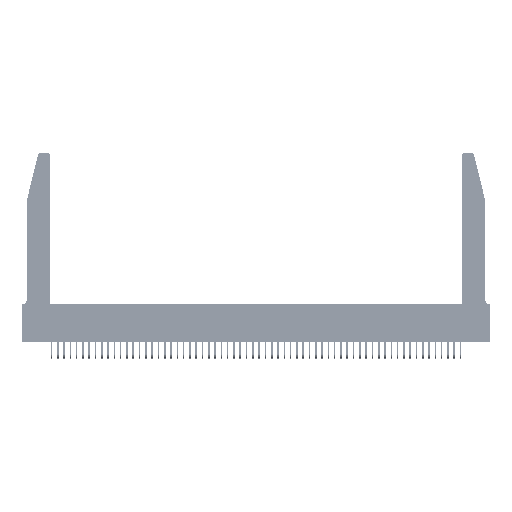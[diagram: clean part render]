
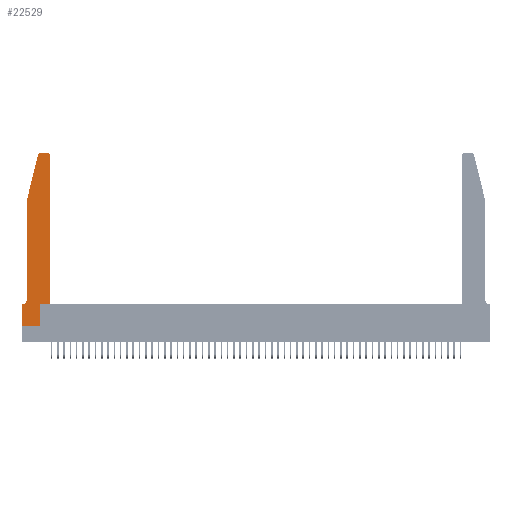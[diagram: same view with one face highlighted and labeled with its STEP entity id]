
A CAD part, top view. The second image highlights one B-rep face of the part: STEP entity #22529.
In plain terms, the highlighted planar face has unit normal (0, 0, 1).
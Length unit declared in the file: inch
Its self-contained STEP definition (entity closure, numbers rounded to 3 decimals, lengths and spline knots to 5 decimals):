
#350 = VECTOR ( 'NONE', #27360, 39.37008 ) ;
#563 = CARTESIAN_POINT ( 'NONE',  ( 0.0755, 0.42, 0.37 ) ) ;
#987 = DIRECTION ( 'NONE',  ( 0., -1., 0. ) ) ;
#1433 = VECTOR ( 'NONE', #987, 39.37008 ) ;
#1503 = CARTESIAN_POINT ( 'NONE',  ( 0.2865, 0., 0.37 ) ) ;
#2649 = CARTESIAN_POINT ( 'NONE',  ( 0., 0., 0.37 ) ) ;
#2734 = CARTESIAN_POINT ( 'NONE',  ( 0.284, 2.72, 0.37 ) ) ;
#3942 = DIRECTION ( 'NONE',  ( 0., 0., 1. ) ) ;
#4755 = ORIENTED_EDGE ( 'NONE', *, *, #19463, .T. ) ;
#5805 = EDGE_CURVE ( 'NONE', #31619, #9378, #43593, .T. ) ;
#7112 = DIRECTION ( 'NONE',  ( 1., 0., 0. ) ) ;
#7385 = EDGE_CURVE ( 'NONE', #28030, #43568, #21678, .T. ) ;
#7864 = EDGE_CURVE ( 'NONE', #11868, #31619, #13019, .T. ) ;
#9285 = LINE ( 'NONE', #33301, #50271 ) ;
#9378 = VERTEX_POINT ( 'NONE', #27630 ) ;
#10865 = CIRCLE ( 'NONE', #11652, 0.03 ) ;
#11652 = AXIS2_PLACEMENT_3D ( 'NONE', #23470, #52870, #27705 ) ;
#11660 = EDGE_CURVE ( 'NONE', #17356, #39878, #17730, .T. ) ;
#11868 = VERTEX_POINT ( 'NONE', #22654 ) ;
#12125 = VECTOR ( 'NONE', #21281, 39.37008 ) ;
#12420 = VECTOR ( 'NONE', #38266, 39.37008 ) ;
#12501 = PLANE ( 'NONE',  #33237 ) ;
#12825 = CARTESIAN_POINT ( 'NONE',  ( 0.0055, 0.42, 0.37 ) ) ;
#12856 = DIRECTION ( 'NONE',  ( 1., 0., 0. ) ) ;
#13019 = LINE ( 'NONE', #30898, #1433 ) ;
#13197 = EDGE_CURVE ( 'NONE', #49335, #43265, #10865, .T. ) ;
#13372 = ORIENTED_EDGE ( 'NONE', *, *, #11660, .T. ) ;
#16410 = VECTOR ( 'NONE', #12856, 39.37008 ) ;
#16465 = CARTESIAN_POINT ( 'NONE',  ( 0.4205, 2.75, 0.37 ) ) ;
#17089 = DIRECTION ( 'NONE',  ( -1., 0., 0. ) ) ;
#17356 = VERTEX_POINT ( 'NONE', #34757 ) ;
#17730 = LINE ( 'NONE', #38128, #16410 ) ;
#18137 = CARTESIAN_POINT ( 'NONE',  ( 0.4505, 0.35, 0.37 ) ) ;
#18162 = LINE ( 'NONE', #18137, #50452 ) ;
#18511 = LINE ( 'NONE', #21687, #52095 ) ;
#18637 = CARTESIAN_POINT ( 'NONE',  ( 0.25487, 2.72718, 0.37 ) ) ;
#18706 = ORIENTED_EDGE ( 'NONE', *, *, #25149, .T. ) ;
#19463 = EDGE_CURVE ( 'NONE', #46100, #38792, #18511, .T. ) ;
#20060 = AXIS2_PLACEMENT_3D ( 'NONE', #2734, #32603, #7112 ) ;
#21048 = CARTESIAN_POINT ( 'NONE',  ( 0., 0.35, 0.37 ) ) ;
#21281 = DIRECTION ( 'NONE',  ( -1., 0., 0. ) ) ;
#21678 = CIRCLE ( 'NONE', #20060, 0.03 ) ;
#21687 = CARTESIAN_POINT ( 'NONE',  ( 0., 0., 0.37 ) ) ;
#22205 = ORIENTED_EDGE ( 'NONE', *, *, #47819, .T. ) ;
#22388 = DIRECTION ( 'NONE',  ( 0., 1., 0. ) ) ;
#22529 = ADVANCED_FACE ( 'NONE', ( #53057 ), #12501, .T. ) ;
#22654 = CARTESIAN_POINT ( 'NONE',  ( 0.0755, 2., 0.37 ) ) ;
#23197 = EDGE_CURVE ( 'NONE', #38792, #17356, #48418, .T. ) ;
#23415 = LINE ( 'NONE', #44891, #12125 ) ;
#23470 = CARTESIAN_POINT ( 'NONE',  ( 0.4205, 2.72, 0.37 ) ) ;
#23704 = LINE ( 'NONE', #25563, #12420 ) ;
#25149 = EDGE_CURVE ( 'NONE', #43265, #28030, #23415, .T. ) ;
#25563 = CARTESIAN_POINT ( 'NONE',  ( 0., 0., 0.37 ) ) ;
#26471 = ORIENTED_EDGE ( 'NONE', *, *, #41336, .T. ) ;
#26591 = CARTESIAN_POINT ( 'NONE',  ( 0., 0.35, 0.37 ) ) ;
#27360 = DIRECTION ( 'NONE',  ( -1., 0., 0. ) ) ;
#27423 = ORIENTED_EDGE ( 'NONE', *, *, #28744, .T. ) ;
#27630 = CARTESIAN_POINT ( 'NONE',  ( 0.0055, 0.35, 0.37 ) ) ;
#27705 = DIRECTION ( 'NONE',  ( 1., 0., 0. ) ) ;
#28030 = VERTEX_POINT ( 'NONE', #54594 ) ;
#28154 = AXIS2_PLACEMENT_3D ( 'NONE', #12825, #42359, #17089 ) ;
#28744 = EDGE_CURVE ( 'NONE', #48209, #46100, #23704, .T. ) ;
#28878 = DIRECTION ( 'NONE',  ( -0.239, -0.971, 0. ) ) ;
#29272 = CARTESIAN_POINT ( 'NONE',  ( 0.2865, 0.35, 0.37 ) ) ;
#30764 = CARTESIAN_POINT ( 'NONE',  ( 0.4505, 0.35, 0.37 ) ) ;
#30898 = CARTESIAN_POINT ( 'NONE',  ( 0.0755, 2., 0.37 ) ) ;
#31619 = VERTEX_POINT ( 'NONE', #563 ) ;
#32603 = DIRECTION ( 'NONE',  ( 0., 0., 1. ) ) ;
#33237 = AXIS2_PLACEMENT_3D ( 'NONE', #21048, #3942, #33758 ) ;
#33301 = CARTESIAN_POINT ( 'NONE',  ( 0.0755, 2., 0.37 ) ) ;
#33758 = DIRECTION ( 'NONE',  ( 1., 0., 0. ) ) ;
#34757 = CARTESIAN_POINT ( 'NONE',  ( 0.2865, 0.35, 0.37 ) ) ;
#36279 = EDGE_CURVE ( 'NONE', #43568, #11868, #9285, .T. ) ;
#37566 = DIRECTION ( 'NONE',  ( 0., 1., 0. ) ) ;
#37717 = ORIENTED_EDGE ( 'NONE', *, *, #7864, .T. ) ;
#37785 = ORIENTED_EDGE ( 'NONE', *, *, #36279, .T. ) ;
#38128 = CARTESIAN_POINT ( 'NONE',  ( 0.4505, 0.35, 0.37 ) ) ;
#38266 = DIRECTION ( 'NONE',  ( 0., -1., 0. ) ) ;
#38483 = DIRECTION ( 'NONE',  ( 1., 0., 0. ) ) ;
#38792 = VERTEX_POINT ( 'NONE', #1503 ) ;
#39560 = CARTESIAN_POINT ( 'NONE',  ( 0.4505, 2.72, 0.37 ) ) ;
#39878 = VERTEX_POINT ( 'NONE', #30764 ) ;
#41336 = EDGE_CURVE ( 'NONE', #39878, #49335, #18162, .T. ) ;
#42008 = ORIENTED_EDGE ( 'NONE', *, *, #23197, .T. ) ;
#42359 = DIRECTION ( 'NONE',  ( 0., 0., -1. ) ) ;
#43265 = VERTEX_POINT ( 'NONE', #16465 ) ;
#43568 = VERTEX_POINT ( 'NONE', #18637 ) ;
#43593 = CIRCLE ( 'NONE', #28154, 0.07 ) ;
#43634 = EDGE_LOOP ( 'NONE', ( #18706, #44659, #37785, #37717, #49162, #22205, #27423, #4755, #42008, #13372, #26471, #51125 ) ) ;
#44086 = CARTESIAN_POINT ( 'NONE',  ( 0.0755, 0.35, 0.37 ) ) ;
#44659 = ORIENTED_EDGE ( 'NONE', *, *, #7385, .T. ) ;
#44891 = CARTESIAN_POINT ( 'NONE',  ( 0.2605, 2.75, 0.37 ) ) ;
#45611 = LINE ( 'NONE', #44086, #350 ) ;
#46100 = VERTEX_POINT ( 'NONE', #2649 ) ;
#47115 = VECTOR ( 'NONE', #37566, 39.37008 ) ;
#47819 = EDGE_CURVE ( 'NONE', #9378, #48209, #45611, .T. ) ;
#48209 = VERTEX_POINT ( 'NONE', #26591 ) ;
#48418 = LINE ( 'NONE', #29272, #47115 ) ;
#49162 = ORIENTED_EDGE ( 'NONE', *, *, #5805, .T. ) ;
#49335 = VERTEX_POINT ( 'NONE', #39560 ) ;
#50271 = VECTOR ( 'NONE', #28878, 39.37008 ) ;
#50452 = VECTOR ( 'NONE', #22388, 39.37008 ) ;
#51125 = ORIENTED_EDGE ( 'NONE', *, *, #13197, .T. ) ;
#52095 = VECTOR ( 'NONE', #38483, 39.37008 ) ;
#52870 = DIRECTION ( 'NONE',  ( 0., 0., 1. ) ) ;
#53057 = FACE_OUTER_BOUND ( 'NONE', #43634, .T. ) ;
#54594 = CARTESIAN_POINT ( 'NONE',  ( 0.284, 2.75, 0.37 ) ) ;
